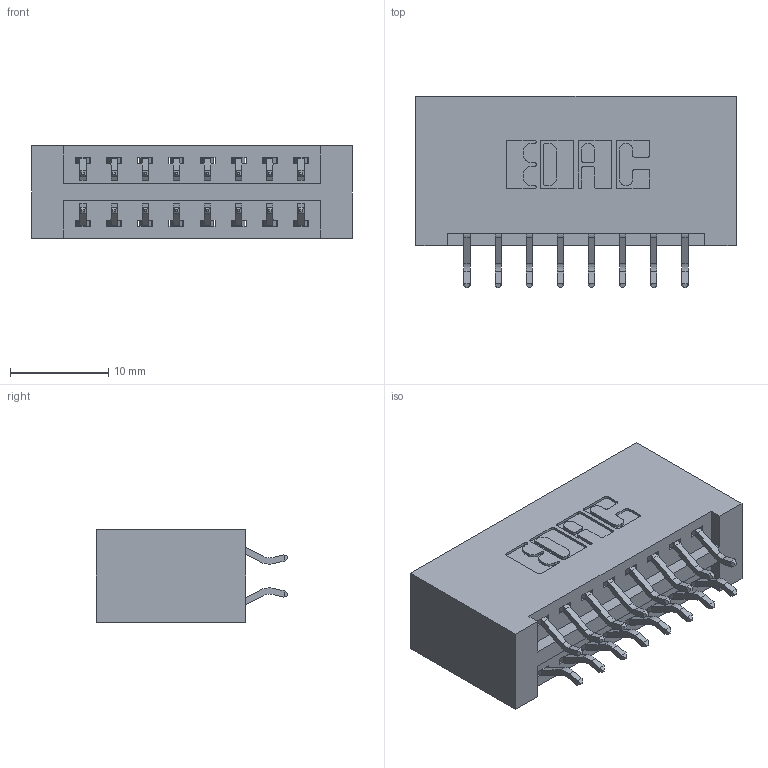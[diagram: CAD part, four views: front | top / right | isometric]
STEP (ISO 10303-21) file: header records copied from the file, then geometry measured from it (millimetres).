
FILE_DESCRIPTION (( 'STEP AP203' ), '1' );
FILE_NAME ('346-016-556-201.STEP', '2022-05-18T16:12:47', ( '' ), ( '' ), 'SwSTEP 2.0', 'SolidWorks 2020', '' );
FILE_SCHEMA (( 'CONFIG_CONTROL_DESIGN' ));
Length unit declared in the file: inch
Products named in the file (3): 346 Part_No Mounting Lugs; 346-016-556-201; 345-292-001_556 Tail
Assembly tree (17 placements, depth 2):
  346-016-556-201
    346 Part_No Mounting Lugs
    345-292-001_556 Tail  x16
Bounding box: 32.64 x 19.57 x 9.4 mm (x, y, z)
Volume: 3491.3 mm3; surface area: 4412.9 mm2
Topology: 17 solids, 17 shells, 1042 faces, 3073 edges, 2026 vertices
Faces by surface type: plane 696, cylinder 346
Entity records: 9741 total; most frequent: CARTESIAN_POINT 1664, ORIENTED_EDGE 1586, DIRECTION 1501, EDGE_CURVE 793, LINE 629, VECTOR 629, VERTEX_POINT 526, AXIS2_PLACEMENT_3D 436
